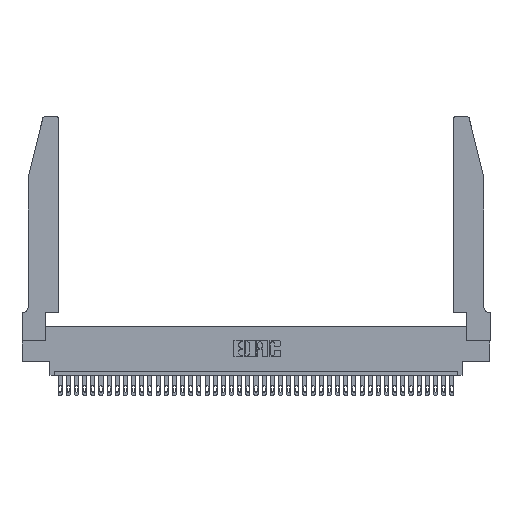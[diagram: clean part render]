
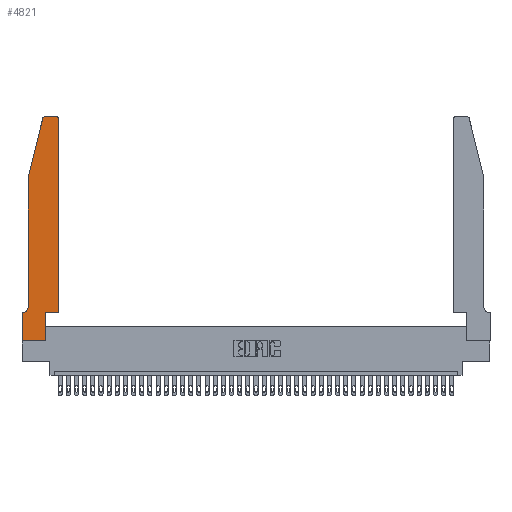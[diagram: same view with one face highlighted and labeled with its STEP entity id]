
A CAD part, top view. The second image highlights one B-rep face of the part: STEP entity #4821.
In plain terms, the highlighted planar face has unit normal (0, 0, 1).
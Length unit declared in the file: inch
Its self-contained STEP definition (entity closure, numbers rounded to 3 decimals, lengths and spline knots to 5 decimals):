
#143 = LINE ( 'NONE', #7516, #9986 ) ;
#512 = VERTEX_POINT ( 'NONE', #14682 ) ;
#694 = VERTEX_POINT ( 'NONE', #24866 ) ;
#1406 = DIRECTION ( 'NONE',  ( 0., -1., 0. ) ) ;
#1724 = CARTESIAN_POINT ( 'NONE',  ( 0.4505, 0.35, 0.37 ) ) ;
#1866 = VECTOR ( 'NONE', #15942, 39.37008 ) ;
#2061 = CARTESIAN_POINT ( 'NONE',  ( 0.2865, 0.35, 0.37 ) ) ;
#2122 = VERTEX_POINT ( 'NONE', #2061 ) ;
#2594 = EDGE_CURVE ( 'NONE', #27120, #33647, #6991, .T. ) ;
#2707 = ORIENTED_EDGE ( 'NONE', *, *, #14837, .T. ) ;
#2711 = DIRECTION ( 'NONE',  ( 0., 0., 1. ) ) ;
#3358 = VERTEX_POINT ( 'NONE', #8338 ) ;
#3470 = CARTESIAN_POINT ( 'NONE',  ( 0.0755, 2., 0.37 ) ) ;
#3582 = ORIENTED_EDGE ( 'NONE', *, *, #28449, .T. ) ;
#3629 = CARTESIAN_POINT ( 'NONE',  ( 0.2605, 2.75, 0.37 ) ) ;
#4820 = ORIENTED_EDGE ( 'NONE', *, *, #16732, .T. ) ;
#4821 = ADVANCED_FACE ( 'NONE', ( #28491 ), #29694, .T. ) ;
#5185 = VERTEX_POINT ( 'NONE', #14168 ) ;
#6225 = DIRECTION ( 'NONE',  ( 1., 0., 0. ) ) ;
#6991 = LINE ( 'NONE', #3470, #26206 ) ;
#7235 = VECTOR ( 'NONE', #35073, 39.37008 ) ;
#7509 = VERTEX_POINT ( 'NONE', #37305 ) ;
#7516 = CARTESIAN_POINT ( 'NONE',  ( 0.2865, 0.35, 0.37 ) ) ;
#7546 = ORIENTED_EDGE ( 'NONE', *, *, #8032, .T. ) ;
#8032 = EDGE_CURVE ( 'NONE', #512, #27120, #12225, .T. ) ;
#8338 = CARTESIAN_POINT ( 'NONE',  ( 0.4205, 2.75, 0.37 ) ) ;
#8589 = CARTESIAN_POINT ( 'NONE',  ( 0.0755, 2., 0.37 ) ) ;
#9945 = CARTESIAN_POINT ( 'NONE',  ( 0., 0.35, 0.37 ) ) ;
#9986 = VECTOR ( 'NONE', #29011, 39.37008 ) ;
#10950 = CARTESIAN_POINT ( 'NONE',  ( 0.284, 2.75, 0.37 ) ) ;
#11006 = LINE ( 'NONE', #1724, #12937 ) ;
#11039 = ORIENTED_EDGE ( 'NONE', *, *, #29110, .T. ) ;
#11405 = CIRCLE ( 'NONE', #40387, 0.03 ) ;
#11409 = DIRECTION ( 'NONE',  ( -1., 0., 0. ) ) ;
#11539 = AXIS2_PLACEMENT_3D ( 'NONE', #21394, #2711, #24582 ) ;
#12213 = DIRECTION ( 'NONE',  ( 1., 0., 0. ) ) ;
#12225 = LINE ( 'NONE', #8589, #1866 ) ;
#12390 = CARTESIAN_POINT ( 'NONE',  ( 0.284, 2.72, 0.37 ) ) ;
#12575 = CARTESIAN_POINT ( 'NONE',  ( 0.2865, 0., 0.37 ) ) ;
#12937 = VECTOR ( 'NONE', #14373, 39.37008 ) ;
#13178 = ORIENTED_EDGE ( 'NONE', *, *, #19806, .T. ) ;
#13421 = ORIENTED_EDGE ( 'NONE', *, *, #37125, .T. ) ;
#14168 = CARTESIAN_POINT ( 'NONE',  ( 0., 0., 0.37 ) ) ;
#14373 = DIRECTION ( 'NONE',  ( 0., 1., 0. ) ) ;
#14574 = CARTESIAN_POINT ( 'NONE',  ( 0.4505, 0.35, 0.37 ) ) ;
#14682 = CARTESIAN_POINT ( 'NONE',  ( 0.25487, 2.72718, 0.37 ) ) ;
#14837 = EDGE_CURVE ( 'NONE', #20992, #2122, #143, .T. ) ;
#15128 = LINE ( 'NONE', #3629, #7235 ) ;
#15572 = DIRECTION ( 'NONE',  ( 0., 0., 1. ) ) ;
#15743 = CIRCLE ( 'NONE', #11539, 0.03 ) ;
#15936 = VECTOR ( 'NONE', #27545, 39.37008 ) ;
#15942 = DIRECTION ( 'NONE',  ( -0.239, -0.971, 0. ) ) ;
#16269 = ORIENTED_EDGE ( 'NONE', *, *, #33433, .T. ) ;
#16482 = VERTEX_POINT ( 'NONE', #9945 ) ;
#16622 = EDGE_CURVE ( 'NONE', #2122, #694, #39419, .T. ) ;
#16732 = EDGE_CURVE ( 'NONE', #32541, #512, #11405, .T. ) ;
#16840 = ORIENTED_EDGE ( 'NONE', *, *, #39298, .T. ) ;
#17686 = LINE ( 'NONE', #34509, #33398 ) ;
#18976 = CARTESIAN_POINT ( 'NONE',  ( 0.0755, 0.35, 0.37 ) ) ;
#19806 = EDGE_CURVE ( 'NONE', #33647, #23873, #39630, .T. ) ;
#20646 = VECTOR ( 'NONE', #25008, 39.37008 ) ;
#20992 = VERTEX_POINT ( 'NONE', #12575 ) ;
#21394 = CARTESIAN_POINT ( 'NONE',  ( 0.4205, 2.72, 0.37 ) ) ;
#21853 = DIRECTION ( 'NONE',  ( 0., 0., 1. ) ) ;
#22295 = LINE ( 'NONE', #18976, #15936 ) ;
#22492 = ORIENTED_EDGE ( 'NONE', *, *, #16622, .T. ) ;
#23065 = AXIS2_PLACEMENT_3D ( 'NONE', #35019, #39984, #11409 ) ;
#23873 = VERTEX_POINT ( 'NONE', #39328 ) ;
#24582 = DIRECTION ( 'NONE',  ( 1., 0., 0. ) ) ;
#24866 = CARTESIAN_POINT ( 'NONE',  ( 0.4505, 0.35, 0.37 ) ) ;
#25008 = DIRECTION ( 'NONE',  ( 0., -1., 0. ) ) ;
#26206 = VECTOR ( 'NONE', #1406, 39.37008 ) ;
#27120 = VERTEX_POINT ( 'NONE', #35939 ) ;
#27545 = DIRECTION ( 'NONE',  ( -1., 0., 0. ) ) ;
#27833 = AXIS2_PLACEMENT_3D ( 'NONE', #34169, #21853, #31634 ) ;
#28073 = CARTESIAN_POINT ( 'NONE',  ( 0., 0., 0.37 ) ) ;
#28449 = EDGE_CURVE ( 'NONE', #16482, #5185, #29053, .T. ) ;
#28491 = FACE_OUTER_BOUND ( 'NONE', #34706, .T. ) ;
#29011 = DIRECTION ( 'NONE',  ( 0., 1., 0. ) ) ;
#29053 = LINE ( 'NONE', #28073, #20646 ) ;
#29110 = EDGE_CURVE ( 'NONE', #5185, #20992, #17686, .T. ) ;
#29694 = PLANE ( 'NONE',  #27833 ) ;
#31634 = DIRECTION ( 'NONE',  ( 1., 0., 0. ) ) ;
#31747 = ORIENTED_EDGE ( 'NONE', *, *, #2594, .T. ) ;
#32541 = VERTEX_POINT ( 'NONE', #10950 ) ;
#32567 = EDGE_CURVE ( 'NONE', #694, #7509, #11006, .T. ) ;
#33398 = VECTOR ( 'NONE', #6225, 39.37008 ) ;
#33433 = EDGE_CURVE ( 'NONE', #3358, #32541, #15128, .T. ) ;
#33514 = ORIENTED_EDGE ( 'NONE', *, *, #32567, .T. ) ;
#33647 = VERTEX_POINT ( 'NONE', #38957 ) ;
#34169 = CARTESIAN_POINT ( 'NONE',  ( 0., 0.35, 0.37 ) ) ;
#34509 = CARTESIAN_POINT ( 'NONE',  ( 0., 0., 0.37 ) ) ;
#34706 = EDGE_LOOP ( 'NONE', ( #16269, #4820, #7546, #31747, #13178, #13421, #3582, #11039, #2707, #22492, #33514, #16840 ) ) ;
#35019 = CARTESIAN_POINT ( 'NONE',  ( 0.0055, 0.42, 0.37 ) ) ;
#35073 = DIRECTION ( 'NONE',  ( -1., 0., 0. ) ) ;
#35939 = CARTESIAN_POINT ( 'NONE',  ( 0.0755, 2., 0.37 ) ) ;
#37125 = EDGE_CURVE ( 'NONE', #23873, #16482, #22295, .T. ) ;
#37305 = CARTESIAN_POINT ( 'NONE',  ( 0.4505, 2.72, 0.37 ) ) ;
#37652 = DIRECTION ( 'NONE',  ( 1., 0., 0. ) ) ;
#38411 = VECTOR ( 'NONE', #12213, 39.37008 ) ;
#38957 = CARTESIAN_POINT ( 'NONE',  ( 0.0755, 0.42, 0.37 ) ) ;
#39298 = EDGE_CURVE ( 'NONE', #7509, #3358, #15743, .T. ) ;
#39328 = CARTESIAN_POINT ( 'NONE',  ( 0.0055, 0.35, 0.37 ) ) ;
#39419 = LINE ( 'NONE', #14574, #38411 ) ;
#39630 = CIRCLE ( 'NONE', #23065, 0.07 ) ;
#39984 = DIRECTION ( 'NONE',  ( 0., 0., -1. ) ) ;
#40387 = AXIS2_PLACEMENT_3D ( 'NONE', #12390, #15572, #37652 ) ;
